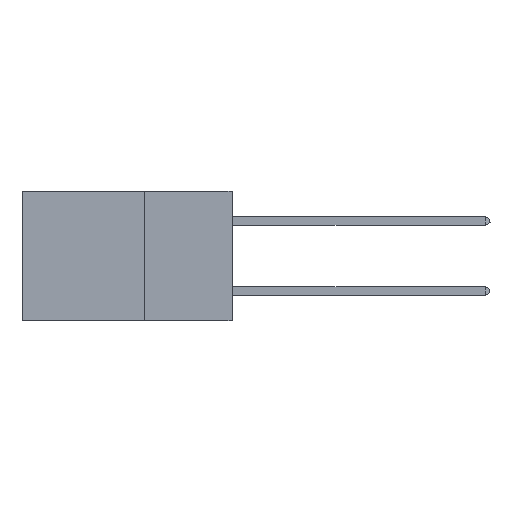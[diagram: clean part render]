
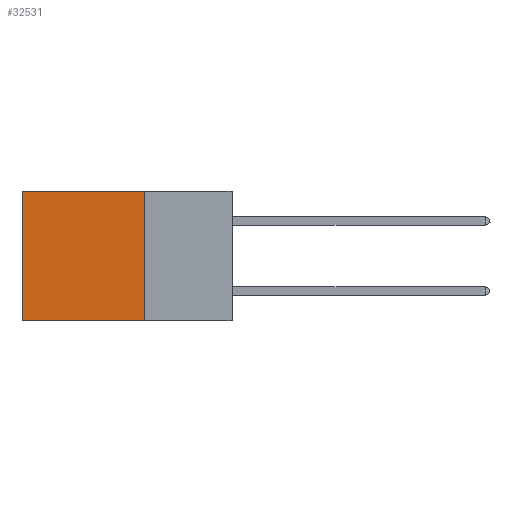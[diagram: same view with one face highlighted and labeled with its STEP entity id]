
A CAD part, left-side view. The second image highlights one B-rep face of the part: STEP entity #32531.
In plain terms, the highlighted planar face has unit normal (-1, 0, 0).
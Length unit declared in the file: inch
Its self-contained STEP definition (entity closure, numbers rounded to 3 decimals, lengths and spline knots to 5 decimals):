
#505 = EDGE_CURVE ( 'NONE', #13406, #31702, #28611, .T. ) ;
#1895 = DIRECTION ( 'NONE',  ( 0., 1., 0. ) ) ;
#2692 = EDGE_LOOP ( 'NONE', ( #15107, #5110, #10215, #26971 ) ) ;
#3526 = AXIS2_PLACEMENT_3D ( 'NONE', #9502, #28182, #28361 ) ;
#3675 = CARTESIAN_POINT ( 'NONE',  ( 0.2875, 0.25, 0. ) ) ;
#5110 = ORIENTED_EDGE ( 'NONE', *, *, #9200, .F. ) ;
#7006 = CARTESIAN_POINT ( 'NONE',  ( 0.2875, 0.25, 0. ) ) ;
#8746 = CARTESIAN_POINT ( 'NONE',  ( 0.2875, 0.6, -0.37 ) ) ;
#8824 = VECTOR ( 'NONE', #31677, 39.37008 ) ;
#9200 = EDGE_CURVE ( 'NONE', #31702, #22198, #12926, .T. ) ;
#9502 = CARTESIAN_POINT ( 'NONE',  ( 0.2875, 0.25, 0. ) ) ;
#10215 = ORIENTED_EDGE ( 'NONE', *, *, #505, .F. ) ;
#12255 = VERTEX_POINT ( 'NONE', #17833 ) ;
#12384 = FACE_OUTER_BOUND ( 'NONE', #2692, .T. ) ;
#12926 = LINE ( 'NONE', #24357, #20401 ) ;
#13406 = VERTEX_POINT ( 'NONE', #3675 ) ;
#14651 = CARTESIAN_POINT ( 'NONE',  ( 0.2875, 0.25, -0.37 ) ) ;
#15107 = ORIENTED_EDGE ( 'NONE', *, *, #22064, .T. ) ;
#15115 = VECTOR ( 'NONE', #35340, 39.37008 ) ;
#17833 = CARTESIAN_POINT ( 'NONE',  ( 0.2875, 0.6, 0. ) ) ;
#20401 = VECTOR ( 'NONE', #1895, 39.37008 ) ;
#21380 = LINE ( 'NONE', #32451, #15115 ) ;
#22064 = EDGE_CURVE ( 'NONE', #12255, #22198, #35564, .T. ) ;
#22198 = VERTEX_POINT ( 'NONE', #8746 ) ;
#23975 = DIRECTION ( 'NONE',  ( 0., 0., -1. ) ) ;
#24357 = CARTESIAN_POINT ( 'NONE',  ( 0.2875, 0.25, -0.37 ) ) ;
#26971 = ORIENTED_EDGE ( 'NONE', *, *, #31465, .T. ) ;
#28182 = DIRECTION ( 'NONE',  ( 1., 0., 0. ) ) ;
#28361 = DIRECTION ( 'NONE',  ( 0., 0., -1. ) ) ;
#28611 = LINE ( 'NONE', #7006, #8824 ) ;
#31465 = EDGE_CURVE ( 'NONE', #13406, #12255, #21380, .T. ) ;
#31538 = VECTOR ( 'NONE', #23975, 39.37008 ) ;
#31677 = DIRECTION ( 'NONE',  ( 0., 0., -1. ) ) ;
#31702 = VERTEX_POINT ( 'NONE', #14651 ) ;
#32451 = CARTESIAN_POINT ( 'NONE',  ( 0.2875, 0.25, 0. ) ) ;
#32531 = ADVANCED_FACE ( 'NONE', ( #12384 ), #34336, .F. ) ;
#34336 = PLANE ( 'NONE',  #3526 ) ;
#35039 = CARTESIAN_POINT ( 'NONE',  ( 0.2875, 0.6, 0. ) ) ;
#35340 = DIRECTION ( 'NONE',  ( 0., 1., 0. ) ) ;
#35564 = LINE ( 'NONE', #35039, #31538 ) ;
